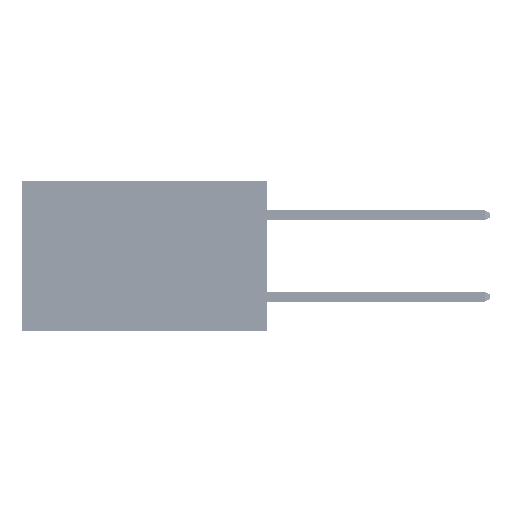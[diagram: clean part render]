
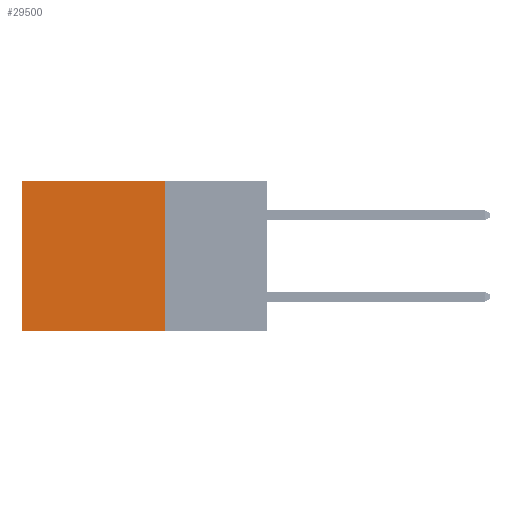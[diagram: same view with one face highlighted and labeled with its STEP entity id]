
A CAD part, left-side view. The second image highlights one B-rep face of the part: STEP entity #29500.
In plain terms, the highlighted planar face has unit normal (-1, 0, 0).
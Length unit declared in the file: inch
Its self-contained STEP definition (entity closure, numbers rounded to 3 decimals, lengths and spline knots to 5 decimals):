
#23 = LINE ( 'NONE', #30231, #3911 ) ;
#985 = DIRECTION ( 'NONE',  ( 0., 1., 0. ) ) ;
#3034 = DIRECTION ( 'NONE',  ( 0., 1., 0. ) ) ;
#3911 = VECTOR ( 'NONE', #985, 39.37008 ) ;
#3996 = DIRECTION ( 'NONE',  ( 1., 0., 0. ) ) ;
#7347 = ORIENTED_EDGE ( 'NONE', *, *, #33402, .F. ) ;
#7394 = FACE_OUTER_BOUND ( 'NONE', #36870, .T. ) ;
#7875 = CARTESIAN_POINT ( 'NONE',  ( 0.2875, 0.25, 0. ) ) ;
#9254 = LINE ( 'NONE', #41403, #26378 ) ;
#10375 = EDGE_CURVE ( 'NONE', #47315, #20598, #35413, .T. ) ;
#15245 = CARTESIAN_POINT ( 'NONE',  ( 0.2875, 0.6, 0. ) ) ;
#18573 = VECTOR ( 'NONE', #3034, 39.37008 ) ;
#20598 = VERTEX_POINT ( 'NONE', #15245 ) ;
#22996 = VECTOR ( 'NONE', #28589, 39.37008 ) ;
#24371 = ORIENTED_EDGE ( 'NONE', *, *, #41949, .T. ) ;
#24418 = EDGE_CURVE ( 'NONE', #28165, #44690, #23, .T. ) ;
#26378 = VECTOR ( 'NONE', #27121, 39.37008 ) ;
#27121 = DIRECTION ( 'NONE',  ( 0., 0., -1. ) ) ;
#28165 = VERTEX_POINT ( 'NONE', #37366 ) ;
#28589 = DIRECTION ( 'NONE',  ( 0., 0., -1. ) ) ;
#29500 = ADVANCED_FACE ( 'NONE', ( #7394 ), #30567, .F. ) ;
#30231 = CARTESIAN_POINT ( 'NONE',  ( 0.2875, 0.25, -0.37 ) ) ;
#30567 = PLANE ( 'NONE',  #41405 ) ;
#32692 = LINE ( 'NONE', #43804, #22996 ) ;
#33402 = EDGE_CURVE ( 'NONE', #47315, #28165, #32692, .T. ) ;
#34689 = CARTESIAN_POINT ( 'NONE',  ( 0.2875, 0.6, -0.37 ) ) ;
#34846 = CARTESIAN_POINT ( 'NONE',  ( 0.2875, 0.25, 0. ) ) ;
#35413 = LINE ( 'NONE', #36125, #18573 ) ;
#36125 = CARTESIAN_POINT ( 'NONE',  ( 0.2875, 0.25, 0. ) ) ;
#36870 = EDGE_LOOP ( 'NONE', ( #24371, #47126, #7347, #38073 ) ) ;
#37096 = DIRECTION ( 'NONE',  ( 0., 0., -1. ) ) ;
#37366 = CARTESIAN_POINT ( 'NONE',  ( 0.2875, 0.25, -0.37 ) ) ;
#38073 = ORIENTED_EDGE ( 'NONE', *, *, #10375, .T. ) ;
#41403 = CARTESIAN_POINT ( 'NONE',  ( 0.2875, 0.6, 0. ) ) ;
#41405 = AXIS2_PLACEMENT_3D ( 'NONE', #7875, #3996, #37096 ) ;
#41949 = EDGE_CURVE ( 'NONE', #20598, #44690, #9254, .T. ) ;
#43804 = CARTESIAN_POINT ( 'NONE',  ( 0.2875, 0.25, 0. ) ) ;
#44690 = VERTEX_POINT ( 'NONE', #34689 ) ;
#47126 = ORIENTED_EDGE ( 'NONE', *, *, #24418, .F. ) ;
#47315 = VERTEX_POINT ( 'NONE', #34846 ) ;
